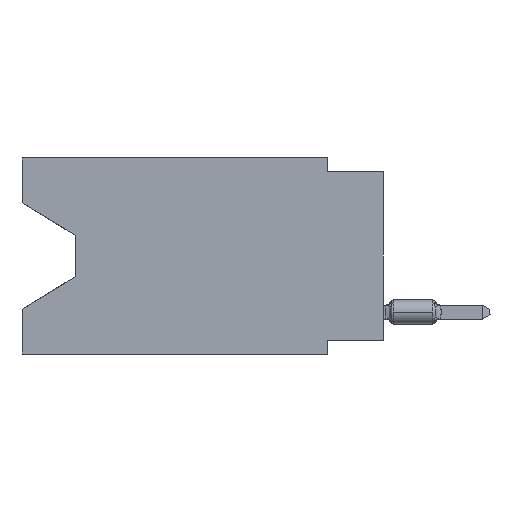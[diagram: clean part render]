
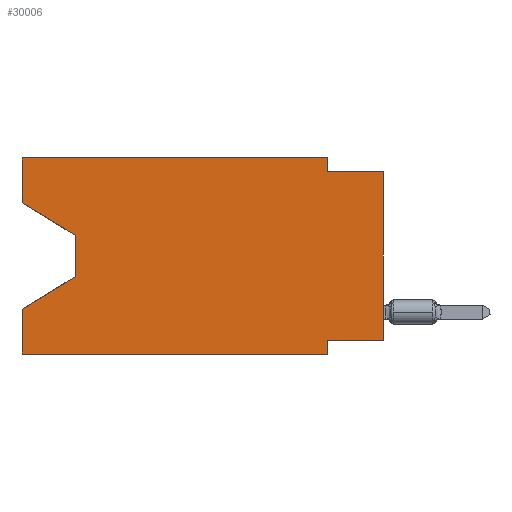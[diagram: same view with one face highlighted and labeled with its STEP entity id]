
A CAD part, left-side view. The second image highlights one B-rep face of the part: STEP entity #30006.
In plain terms, the highlighted planar face has unit normal (-1, 0, 0).
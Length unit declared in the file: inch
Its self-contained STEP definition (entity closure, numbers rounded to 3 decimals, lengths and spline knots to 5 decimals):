
#946 = VERTEX_POINT ( 'NONE', #34157 ) ;
#1362 = DIRECTION ( 'NONE',  ( 0., -0.855, -0.519 ) ) ;
#1761 = CARTESIAN_POINT ( 'NONE',  ( 0., 0.1, -0.35 ) ) ;
#2586 = ORIENTED_EDGE ( 'NONE', *, *, #60939, .F. ) ;
#2711 = VECTOR ( 'NONE', #7355, 39.37008 ) ;
#3131 = EDGE_CURVE ( 'NONE', #46036, #67769, #47111, .T. ) ;
#3605 = CARTESIAN_POINT ( 'NONE',  ( 0., 0.645, 0. ) ) ;
#4478 = DIRECTION ( 'NONE',  ( 0., 0., 1. ) ) ;
#6147 = CARTESIAN_POINT ( 'NONE',  ( 0., 0.55, -0.138 ) ) ;
#7355 = DIRECTION ( 'NONE',  ( 0., 0., -1. ) ) ;
#7571 = CARTESIAN_POINT ( 'NONE',  ( 0., 0.1, -0.325 ) ) ;
#8355 = VERTEX_POINT ( 'NONE', #65516 ) ;
#8859 = CARTESIAN_POINT ( 'NONE',  ( 0., 0.55, -0.138 ) ) ;
#9031 = CARTESIAN_POINT ( 'NONE',  ( 0., 0.55, -0.212 ) ) ;
#11170 = VECTOR ( 'NONE', #17545, 39.37008 ) ;
#12252 = LINE ( 'NONE', #33904, #55276 ) ;
#12871 = VECTOR ( 'NONE', #56381, 39.37008 ) ;
#13370 = CARTESIAN_POINT ( 'NONE',  ( 0., 0.645, -0.35 ) ) ;
#13599 = CARTESIAN_POINT ( 'NONE',  ( 0., 0.645, 0. ) ) ;
#15384 = EDGE_CURVE ( 'NONE', #18083, #33922, #67111, .T. ) ;
#15615 = CARTESIAN_POINT ( 'NONE',  ( 0., 0.55, -0.212 ) ) ;
#16318 = ORIENTED_EDGE ( 'NONE', *, *, #22633, .T. ) ;
#17155 = LINE ( 'NONE', #1761, #11170 ) ;
#17545 = DIRECTION ( 'NONE',  ( 0., 0., -1. ) ) ;
#17714 = VERTEX_POINT ( 'NONE', #40290 ) ;
#17956 = DIRECTION ( 'NONE',  ( 0., 1., 0. ) ) ;
#18083 = VERTEX_POINT ( 'NONE', #41257 ) ;
#19347 = CARTESIAN_POINT ( 'NONE',  ( 0., 0.1, -0.35 ) ) ;
#19371 = ORIENTED_EDGE ( 'NONE', *, *, #25439, .T. ) ;
#20179 = VECTOR ( 'NONE', #45466, 39.37008 ) ;
#20525 = DIRECTION ( 'NONE',  ( 0., 0.855, -0.519 ) ) ;
#20839 = ORIENTED_EDGE ( 'NONE', *, *, #64235, .F. ) ;
#22633 = EDGE_CURVE ( 'NONE', #55508, #46036, #36105, .T. ) ;
#23692 = VECTOR ( 'NONE', #67959, 39.37008 ) ;
#25439 = EDGE_CURVE ( 'NONE', #17714, #946, #46852, .T. ) ;
#27219 = ORIENTED_EDGE ( 'NONE', *, *, #39931, .T. ) ;
#27673 = CARTESIAN_POINT ( 'NONE',  ( 0., 0.645, -0.08025 ) ) ;
#28044 = ORIENTED_EDGE ( 'NONE', *, *, #15384, .F. ) ;
#28115 = EDGE_LOOP ( 'NONE', ( #27219, #16318, #48276, #59906, #64070, #46681, #20839, #19371, #2586, #65383, #32408, #28044 ) ) ;
#29416 = VERTEX_POINT ( 'NONE', #40548 ) ;
#30006 = ADVANCED_FACE ( 'NONE', ( #38299 ), #54065, .F. ) ;
#31178 = EDGE_CURVE ( 'NONE', #8355, #67769, #33919, .T. ) ;
#32408 = ORIENTED_EDGE ( 'NONE', *, *, #46844, .F. ) ;
#32490 = EDGE_CURVE ( 'NONE', #8355, #50403, #40283, .T. ) ;
#32871 = VECTOR ( 'NONE', #20525, 39.37008 ) ;
#33904 = CARTESIAN_POINT ( 'NONE',  ( 0., 0., -0.025 ) ) ;
#33919 = LINE ( 'NONE', #54933, #59626 ) ;
#33922 = VERTEX_POINT ( 'NONE', #3605 ) ;
#34157 = CARTESIAN_POINT ( 'NONE',  ( 0., 0., -0.025 ) ) ;
#35060 = CARTESIAN_POINT ( 'NONE',  ( 0., 0.645, -0.26975 ) ) ;
#36105 = LINE ( 'NONE', #8859, #23692 ) ;
#36463 = CARTESIAN_POINT ( 'NONE',  ( 0., 0.1, 0. ) ) ;
#38299 = FACE_OUTER_BOUND ( 'NONE', #28115, .T. ) ;
#38679 = DIRECTION ( 'NONE',  ( 1., 0., 0. ) ) ;
#38963 = CARTESIAN_POINT ( 'NONE',  ( 0., 0., -0.325 ) ) ;
#39323 = VECTOR ( 'NONE', #17956, 39.37008 ) ;
#39931 = EDGE_CURVE ( 'NONE', #18083, #55508, #69029, .T. ) ;
#40283 = LINE ( 'NONE', #13370, #12871 ) ;
#40290 = CARTESIAN_POINT ( 'NONE',  ( 0., 0., -0.325 ) ) ;
#40548 = CARTESIAN_POINT ( 'NONE',  ( 0., 0.1, -0.025 ) ) ;
#41257 = CARTESIAN_POINT ( 'NONE',  ( 0., 0.645, -0.08025 ) ) ;
#43097 = VECTOR ( 'NONE', #44223, 39.37008 ) ;
#43509 = CARTESIAN_POINT ( 'NONE',  ( 0., 0.645, 0. ) ) ;
#44223 = DIRECTION ( 'NONE',  ( 0., -1., 0. ) ) ;
#44571 = LINE ( 'NONE', #38963, #39323 ) ;
#45466 = DIRECTION ( 'NONE',  ( 0., 0., 1. ) ) ;
#46036 = VERTEX_POINT ( 'NONE', #9031 ) ;
#46286 = VERTEX_POINT ( 'NONE', #7571 ) ;
#46681 = ORIENTED_EDGE ( 'NONE', *, *, #55004, .F. ) ;
#46844 = EDGE_CURVE ( 'NONE', #33922, #58137, #58912, .T. ) ;
#46852 = LINE ( 'NONE', #67467, #49754 ) ;
#47111 = LINE ( 'NONE', #15615, #32871 ) ;
#48276 = ORIENTED_EDGE ( 'NONE', *, *, #3131, .T. ) ;
#49754 = VECTOR ( 'NONE', #4478, 39.37008 ) ;
#50403 = VERTEX_POINT ( 'NONE', #19347 ) ;
#50982 = VECTOR ( 'NONE', #1362, 39.37008 ) ;
#54065 = PLANE ( 'NONE',  #61730 ) ;
#54455 = DIRECTION ( 'NONE',  ( 0., 0., -1. ) ) ;
#54599 = DIRECTION ( 'NONE',  ( 0., -1., 0. ) ) ;
#54933 = CARTESIAN_POINT ( 'NONE',  ( 0., 0.645, 0. ) ) ;
#54948 = LINE ( 'NONE', #65770, #2711 ) ;
#55004 = EDGE_CURVE ( 'NONE', #46286, #50403, #17155, .T. ) ;
#55276 = VECTOR ( 'NONE', #54599, 39.37008 ) ;
#55287 = DIRECTION ( 'NONE',  ( 0., 0., 1. ) ) ;
#55508 = VERTEX_POINT ( 'NONE', #6147 ) ;
#56381 = DIRECTION ( 'NONE',  ( 0., -1., 0. ) ) ;
#58137 = VERTEX_POINT ( 'NONE', #36463 ) ;
#58912 = LINE ( 'NONE', #43509, #43097 ) ;
#59626 = VECTOR ( 'NONE', #55287, 39.37008 ) ;
#59906 = ORIENTED_EDGE ( 'NONE', *, *, #31178, .F. ) ;
#60939 = EDGE_CURVE ( 'NONE', #29416, #946, #12252, .T. ) ;
#61730 = AXIS2_PLACEMENT_3D ( 'NONE', #65608, #38679, #54455 ) ;
#64070 = ORIENTED_EDGE ( 'NONE', *, *, #32490, .T. ) ;
#64235 = EDGE_CURVE ( 'NONE', #17714, #46286, #44571, .T. ) ;
#65383 = ORIENTED_EDGE ( 'NONE', *, *, #68222, .F. ) ;
#65516 = CARTESIAN_POINT ( 'NONE',  ( 0., 0.645, -0.35 ) ) ;
#65608 = CARTESIAN_POINT ( 'NONE',  ( 0., 0.645, 0. ) ) ;
#65770 = CARTESIAN_POINT ( 'NONE',  ( 0., 0.1, 0. ) ) ;
#67111 = LINE ( 'NONE', #13599, #20179 ) ;
#67467 = CARTESIAN_POINT ( 'NONE',  ( 0., 0., 0. ) ) ;
#67769 = VERTEX_POINT ( 'NONE', #35060 ) ;
#67959 = DIRECTION ( 'NONE',  ( 0., 0., -1. ) ) ;
#68222 = EDGE_CURVE ( 'NONE', #58137, #29416, #54948, .T. ) ;
#69029 = LINE ( 'NONE', #27673, #50982 ) ;
